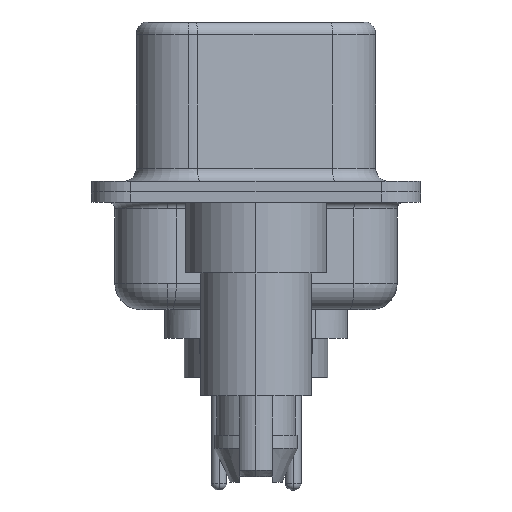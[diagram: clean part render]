
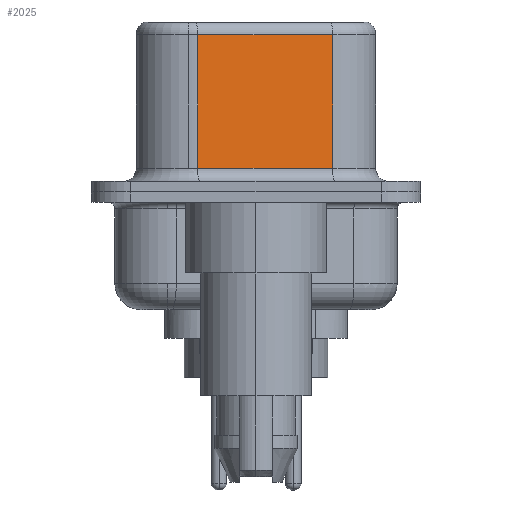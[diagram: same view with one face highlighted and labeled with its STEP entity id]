
A CAD part, left-side view. The second image highlights one B-rep face of the part: STEP entity #2025.
In plain terms, the highlighted planar face has unit normal (-0.985, -0.174, 0).
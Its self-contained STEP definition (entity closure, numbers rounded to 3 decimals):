
#235 = CARTESIAN_POINT ( 'NONE',  ( 3.655, 2.233, 6.52 ) ) ;
#492 = CARTESIAN_POINT ( 'NONE',  ( 3.655, 2.233, 0.9 ) ) ;
#830 = LINE ( 'NONE', #14001, #11004 ) ;
#860 = CARTESIAN_POINT ( 'NONE',  ( 4.565, -2.927, 0.9 ) ) ;
#1413 = PLANE ( 'NONE',  #12493 ) ;
#2025 = ADVANCED_FACE ( 'NONE', ( #2099 ), #1413, .F. ) ;
#2099 = FACE_OUTER_BOUND ( 'NONE', #3713, .T. ) ;
#2735 = LINE ( 'NONE', #860, #17219 ) ;
#2875 = VECTOR ( 'NONE', #10985, 1000. ) ;
#3189 = EDGE_CURVE ( 'NONE', #12773, #15219, #3527, .T. ) ;
#3197 = ORIENTED_EDGE ( 'NONE', *, *, #11644, .T. ) ;
#3527 = LINE ( 'NONE', #235, #11415 ) ;
#3713 = EDGE_LOOP ( 'NONE', ( #16984, #3197, #16688, #17021 ) ) ;
#5332 = CARTESIAN_POINT ( 'NONE',  ( 4.565, -2.927, 6.02 ) ) ;
#5947 = CARTESIAN_POINT ( 'NONE',  ( 4.565, -2.927, 0.9 ) ) ;
#6235 = DIRECTION ( 'NONE',  ( 0.174, -0.985, 0. ) ) ;
#6578 = LINE ( 'NONE', #5332, #2875 ) ;
#8025 = CARTESIAN_POINT ( 'NONE',  ( 4.565, -2.927, 6.02 ) ) ;
#8437 = EDGE_CURVE ( 'NONE', #15219, #15962, #2735, .T. ) ;
#8598 = DIRECTION ( 'NONE',  ( 0., 0., -1. ) ) ;
#8695 = DIRECTION ( 'NONE',  ( 0.985, 0.174, 0. ) ) ;
#8782 = DIRECTION ( 'NONE',  ( -0.174, 0.985, 0. ) ) ;
#9370 = EDGE_CURVE ( 'NONE', #11557, #15962, #830, .T. ) ;
#9845 = DIRECTION ( 'NONE',  ( 0., 0., -1. ) ) ;
#10985 = DIRECTION ( 'NONE',  ( -0.174, 0.985, 0. ) ) ;
#11004 = VECTOR ( 'NONE', #9845, 1000. ) ;
#11415 = VECTOR ( 'NONE', #8598, 1000. ) ;
#11557 = VERTEX_POINT ( 'NONE', #8025 ) ;
#11644 = EDGE_CURVE ( 'NONE', #11557, #12773, #6578, .T. ) ;
#12493 = AXIS2_PLACEMENT_3D ( 'NONE', #17932, #8695, #8782 ) ;
#12773 = VERTEX_POINT ( 'NONE', #17130 ) ;
#14001 = CARTESIAN_POINT ( 'NONE',  ( 4.565, -2.927, 6.52 ) ) ;
#15219 = VERTEX_POINT ( 'NONE', #492 ) ;
#15962 = VERTEX_POINT ( 'NONE', #5947 ) ;
#16688 = ORIENTED_EDGE ( 'NONE', *, *, #3189, .T. ) ;
#16984 = ORIENTED_EDGE ( 'NONE', *, *, #9370, .F. ) ;
#17021 = ORIENTED_EDGE ( 'NONE', *, *, #8437, .T. ) ;
#17130 = CARTESIAN_POINT ( 'NONE',  ( 3.655, 2.233, 6.02 ) ) ;
#17219 = VECTOR ( 'NONE', #6235, 1000. ) ;
#17932 = CARTESIAN_POINT ( 'NONE',  ( 4.565, -2.927, 6.52 ) ) ;
